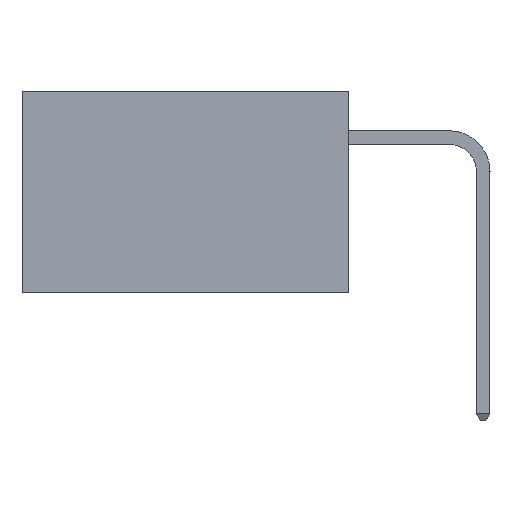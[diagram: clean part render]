
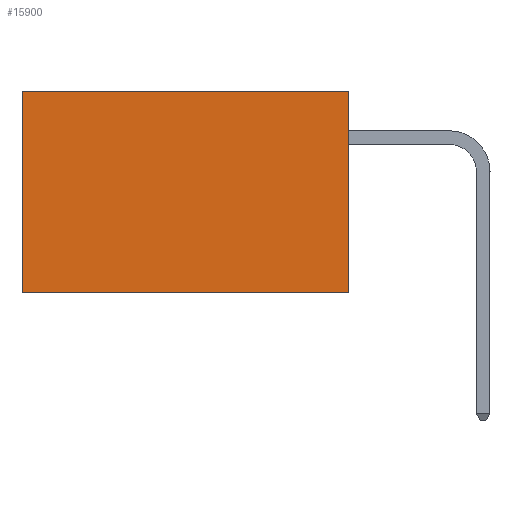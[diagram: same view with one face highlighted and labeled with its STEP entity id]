
A CAD part, left-side view. The second image highlights one B-rep face of the part: STEP entity #15900.
In plain terms, the highlighted planar face has unit normal (-1, 0, 0).
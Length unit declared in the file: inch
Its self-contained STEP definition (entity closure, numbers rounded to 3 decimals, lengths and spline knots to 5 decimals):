
#481 = CARTESIAN_POINT ( 'NONE',  ( 0.2875, 0., -0.37 ) ) ;
#907 = CARTESIAN_POINT ( 'NONE',  ( 0.2875, 0.6, -0.37 ) ) ;
#5102 = VECTOR ( 'NONE', #20682, 39.37008 ) ;
#6005 = LINE ( 'NONE', #11745, #5102 ) ;
#9628 = CARTESIAN_POINT ( 'NONE',  ( 0.2875, 0.6, 0. ) ) ;
#11652 = AXIS2_PLACEMENT_3D ( 'NONE', #15137, #35481, #18128 ) ;
#11745 = CARTESIAN_POINT ( 'NONE',  ( 0.2875, 0., 0. ) ) ;
#11858 = DIRECTION ( 'NONE',  ( 0., 0., -1. ) ) ;
#12562 = DIRECTION ( 'NONE',  ( 0., 0., -1. ) ) ;
#13944 = EDGE_CURVE ( 'NONE', #35845, #22951, #23322, .T. ) ;
#15137 = CARTESIAN_POINT ( 'NONE',  ( 0.2875, 0., 0. ) ) ;
#15885 = VECTOR ( 'NONE', #11858, 39.37008 ) ;
#15900 = ADVANCED_FACE ( 'NONE', ( #27556 ), #29705, .F. ) ;
#18128 = DIRECTION ( 'NONE',  ( 0., 0., -1. ) ) ;
#19967 = ORIENTED_EDGE ( 'NONE', *, *, #30991, .F. ) ;
#20242 = ORIENTED_EDGE ( 'NONE', *, *, #36684, .T. ) ;
#20682 = DIRECTION ( 'NONE',  ( 0., 1., 0. ) ) ;
#22513 = CARTESIAN_POINT ( 'NONE',  ( 0.2875, 0., -0.37 ) ) ;
#22911 = CARTESIAN_POINT ( 'NONE',  ( 0.2875, 0., 0. ) ) ;
#22951 = VERTEX_POINT ( 'NONE', #907 ) ;
#23204 = VERTEX_POINT ( 'NONE', #36660 ) ;
#23322 = LINE ( 'NONE', #481, #30979 ) ;
#25943 = LINE ( 'NONE', #9628, #32731 ) ;
#27251 = ORIENTED_EDGE ( 'NONE', *, *, #13944, .F. ) ;
#27556 = FACE_OUTER_BOUND ( 'NONE', #28168, .T. ) ;
#28168 = EDGE_LOOP ( 'NONE', ( #34584, #27251, #19967, #20242 ) ) ;
#29370 = CARTESIAN_POINT ( 'NONE',  ( 0.2875, 0., 0. ) ) ;
#29454 = DIRECTION ( 'NONE',  ( 0., 1., 0. ) ) ;
#29705 = PLANE ( 'NONE',  #11652 ) ;
#30979 = VECTOR ( 'NONE', #29454, 39.37008 ) ;
#30991 = EDGE_CURVE ( 'NONE', #31432, #35845, #31389, .T. ) ;
#31389 = LINE ( 'NONE', #29370, #15885 ) ;
#31432 = VERTEX_POINT ( 'NONE', #22911 ) ;
#31790 = EDGE_CURVE ( 'NONE', #23204, #22951, #25943, .T. ) ;
#32731 = VECTOR ( 'NONE', #12562, 39.37008 ) ;
#34584 = ORIENTED_EDGE ( 'NONE', *, *, #31790, .T. ) ;
#35481 = DIRECTION ( 'NONE',  ( 1., 0., 0. ) ) ;
#35845 = VERTEX_POINT ( 'NONE', #22513 ) ;
#36660 = CARTESIAN_POINT ( 'NONE',  ( 0.2875, 0.6, 0. ) ) ;
#36684 = EDGE_CURVE ( 'NONE', #31432, #23204, #6005, .T. ) ;
